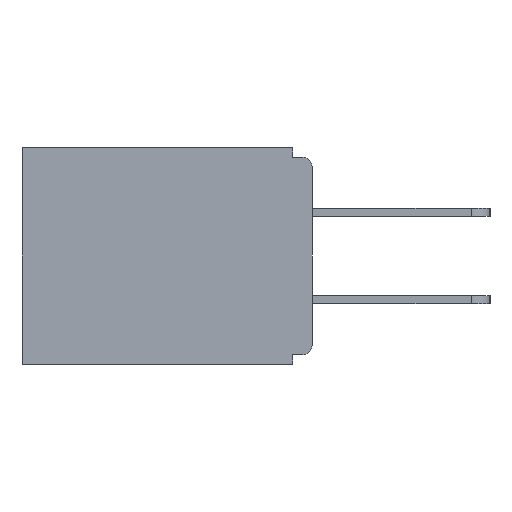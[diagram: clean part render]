
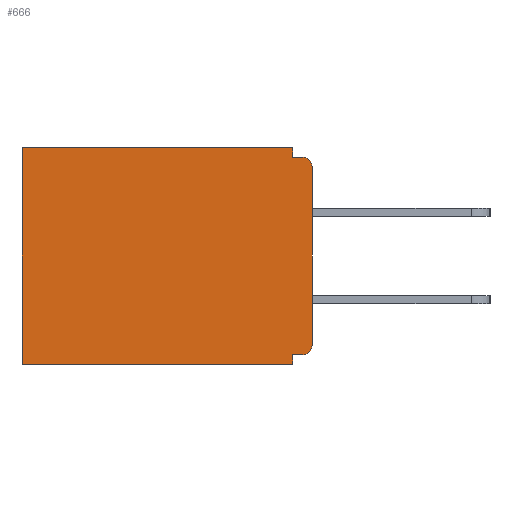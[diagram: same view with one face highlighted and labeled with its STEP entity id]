
A CAD part, left-side view. The second image highlights one B-rep face of the part: STEP entity #666.
In plain terms, the highlighted planar face has unit normal (-1, 0, 0).
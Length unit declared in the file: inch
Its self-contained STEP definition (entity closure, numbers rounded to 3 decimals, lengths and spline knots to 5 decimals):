
#143 = ORIENTED_EDGE ( 'NONE', *, *, #24119, .F. ) ;
#396 = CARTESIAN_POINT ( 'NONE',  ( 0.298, 0.46, 0. ) ) ;
#643 = LINE ( 'NONE', #3961, #1647 ) ;
#666 = ADVANCED_FACE ( 'NONE', ( #16169 ), #26962, .F. ) ;
#828 = CARTESIAN_POINT ( 'NONE',  ( 0.298, 0.015, -0.328 ) ) ;
#1117 = CARTESIAN_POINT ( 'NONE',  ( 0.298, 0., -0.313 ) ) ;
#1128 = DIRECTION ( 'NONE',  ( 1., 0., 0. ) ) ;
#1586 = CARTESIAN_POINT ( 'NONE',  ( 0.298, 0.015, -0.015 ) ) ;
#1637 = ORIENTED_EDGE ( 'NONE', *, *, #12049, .F. ) ;
#1647 = VECTOR ( 'NONE', #27060, 39.37008 ) ;
#1886 = ORIENTED_EDGE ( 'NONE', *, *, #14584, .F. ) ;
#2177 = VERTEX_POINT ( 'NONE', #9847 ) ;
#2915 = CARTESIAN_POINT ( 'NONE',  ( 0.298, 0., 0. ) ) ;
#3728 = VERTEX_POINT ( 'NONE', #14640 ) ;
#3774 = EDGE_CURVE ( 'NONE', #27280, #12480, #6138, .T. ) ;
#3961 = CARTESIAN_POINT ( 'NONE',  ( 0.298, 0.031, -0.343 ) ) ;
#4580 = DIRECTION ( 'NONE',  ( -1., 0., 0. ) ) ;
#4658 = LINE ( 'NONE', #25078, #26257 ) ;
#5272 = CARTESIAN_POINT ( 'NONE',  ( 0.298, 0.031, 0. ) ) ;
#5635 = DIRECTION ( 'NONE',  ( 0., 1., 0. ) ) ;
#5657 = DIRECTION ( 'NONE',  ( 0., 0., -1. ) ) ;
#5841 = ORIENTED_EDGE ( 'NONE', *, *, #18718, .T. ) ;
#6006 = CIRCLE ( 'NONE', #15082, 0.015 ) ;
#6138 = LINE ( 'NONE', #23731, #6833 ) ;
#6182 = ORIENTED_EDGE ( 'NONE', *, *, #21575, .T. ) ;
#6325 = DIRECTION ( 'NONE',  ( 0., -1., 0. ) ) ;
#6459 = VERTEX_POINT ( 'NONE', #828 ) ;
#6460 = ORIENTED_EDGE ( 'NONE', *, *, #23342, .T. ) ;
#6741 = CARTESIAN_POINT ( 'NONE',  ( 0.298, 0.031, -0.015 ) ) ;
#6833 = VECTOR ( 'NONE', #19340, 39.37008 ) ;
#7442 = LINE ( 'NONE', #19557, #16533 ) ;
#8185 = CARTESIAN_POINT ( 'NONE',  ( 0.298, 0.46, 0. ) ) ;
#8273 = CARTESIAN_POINT ( 'NONE',  ( 0.298, 0., -0.343 ) ) ;
#9244 = ORIENTED_EDGE ( 'NONE', *, *, #18915, .F. ) ;
#9847 = CARTESIAN_POINT ( 'NONE',  ( 0.298, 0.031, -0.343 ) ) ;
#9890 = LINE ( 'NONE', #8185, #25086 ) ;
#11652 = AXIS2_PLACEMENT_3D ( 'NONE', #15502, #4580, #21668 ) ;
#12049 = EDGE_CURVE ( 'NONE', #15759, #21035, #4658, .T. ) ;
#12432 = EDGE_CURVE ( 'NONE', #27280, #25430, #6006, .T. ) ;
#12480 = VERTEX_POINT ( 'NONE', #1117 ) ;
#13199 = EDGE_CURVE ( 'NONE', #6459, #3728, #23863, .T. ) ;
#13832 = DIRECTION ( 'NONE',  ( 0., 0., -1. ) ) ;
#13880 = EDGE_LOOP ( 'NONE', ( #21390, #9244, #1637, #5841, #6182, #1886, #143, #19178, #6460, #25613 ) ) ;
#14584 = EDGE_CURVE ( 'NONE', #2177, #14846, #25901, .T. ) ;
#14640 = CARTESIAN_POINT ( 'NONE',  ( 0.298, 0.031, -0.328 ) ) ;
#14846 = VERTEX_POINT ( 'NONE', #22385 ) ;
#15082 = AXIS2_PLACEMENT_3D ( 'NONE', #24798, #26668, #24885 ) ;
#15502 = CARTESIAN_POINT ( 'NONE',  ( 0.298, 0.015, -0.313 ) ) ;
#15759 = VERTEX_POINT ( 'NONE', #5272 ) ;
#16169 = FACE_OUTER_BOUND ( 'NONE', #13880, .T. ) ;
#16533 = VECTOR ( 'NONE', #6325, 39.37008 ) ;
#16987 = VERTEX_POINT ( 'NONE', #396 ) ;
#18292 = CARTESIAN_POINT ( 'NONE',  ( 0.298, 0., -0.328 ) ) ;
#18718 = EDGE_CURVE ( 'NONE', #15759, #16987, #26353, .T. ) ;
#18915 = EDGE_CURVE ( 'NONE', #21035, #25430, #7442, .T. ) ;
#19178 = ORIENTED_EDGE ( 'NONE', *, *, #13199, .F. ) ;
#19340 = DIRECTION ( 'NONE',  ( 0., 0., -1. ) ) ;
#19557 = CARTESIAN_POINT ( 'NONE',  ( 0.298, 0., -0.015 ) ) ;
#19734 = DIRECTION ( 'NONE',  ( 0., 0., -1. ) ) ;
#20677 = DIRECTION ( 'NONE',  ( 0., 1., 0. ) ) ;
#21035 = VERTEX_POINT ( 'NONE', #6741 ) ;
#21390 = ORIENTED_EDGE ( 'NONE', *, *, #12432, .T. ) ;
#21470 = VECTOR ( 'NONE', #20677, 39.37008 ) ;
#21575 = EDGE_CURVE ( 'NONE', #16987, #14846, #9890, .T. ) ;
#21668 = DIRECTION ( 'NONE',  ( 0., 0., -1. ) ) ;
#21849 = DIRECTION ( 'NONE',  ( 0., 1., 0. ) ) ;
#22385 = CARTESIAN_POINT ( 'NONE',  ( 0.298, 0.46, -0.343 ) ) ;
#22642 = VECTOR ( 'NONE', #5635, 39.37008 ) ;
#22803 = CARTESIAN_POINT ( 'NONE',  ( 0.298, 0., 0. ) ) ;
#23203 = VECTOR ( 'NONE', #21849, 39.37008 ) ;
#23342 = EDGE_CURVE ( 'NONE', #6459, #12480, #26993, .T. ) ;
#23731 = CARTESIAN_POINT ( 'NONE',  ( 0.298, 0., 0. ) ) ;
#23789 = AXIS2_PLACEMENT_3D ( 'NONE', #2915, #1128, #13832 ) ;
#23863 = LINE ( 'NONE', #18292, #21470 ) ;
#24119 = EDGE_CURVE ( 'NONE', #3728, #2177, #643, .T. ) ;
#24341 = CARTESIAN_POINT ( 'NONE',  ( 0.298, 0., -0.03 ) ) ;
#24798 = CARTESIAN_POINT ( 'NONE',  ( 0.298, 0.015, -0.03 ) ) ;
#24885 = DIRECTION ( 'NONE',  ( 0., 0., -1. ) ) ;
#25078 = CARTESIAN_POINT ( 'NONE',  ( 0.298, 0.031, -0.343 ) ) ;
#25086 = VECTOR ( 'NONE', #19734, 39.37008 ) ;
#25430 = VERTEX_POINT ( 'NONE', #1586 ) ;
#25613 = ORIENTED_EDGE ( 'NONE', *, *, #3774, .F. ) ;
#25901 = LINE ( 'NONE', #8273, #23203 ) ;
#26257 = VECTOR ( 'NONE', #5657, 39.37008 ) ;
#26353 = LINE ( 'NONE', #22803, #22642 ) ;
#26668 = DIRECTION ( 'NONE',  ( -1., 0., 0. ) ) ;
#26962 = PLANE ( 'NONE',  #23789 ) ;
#26993 = CIRCLE ( 'NONE', #11652, 0.015 ) ;
#27060 = DIRECTION ( 'NONE',  ( 0., 0., -1. ) ) ;
#27280 = VERTEX_POINT ( 'NONE', #24341 ) ;
